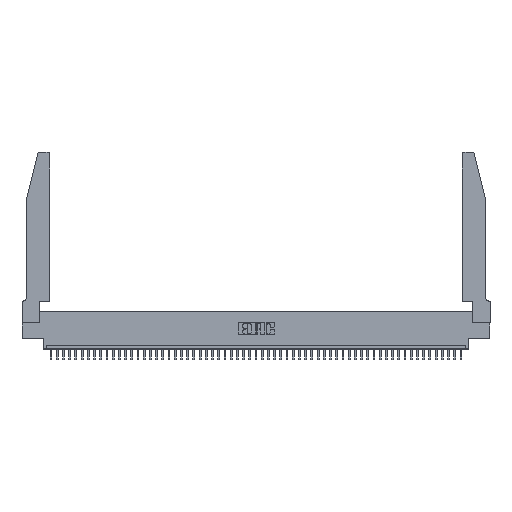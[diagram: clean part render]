
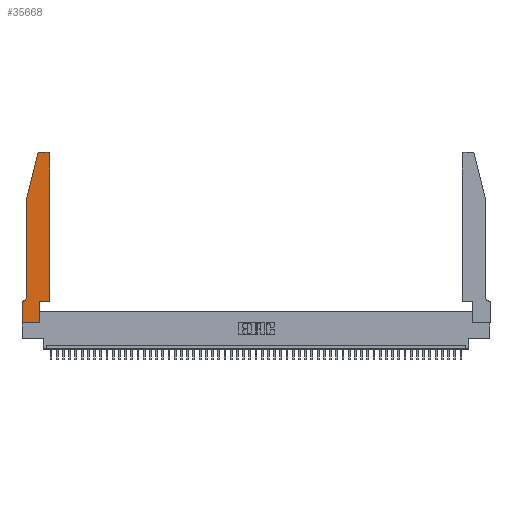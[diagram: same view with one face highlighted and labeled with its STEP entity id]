
A CAD part, top view. The second image highlights one B-rep face of the part: STEP entity #35668.
In plain terms, the highlighted planar face has unit normal (0, 0, 1).
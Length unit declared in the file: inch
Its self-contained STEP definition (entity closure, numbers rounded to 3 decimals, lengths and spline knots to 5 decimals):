
#62 = ORIENTED_EDGE ( 'NONE', *, *, #50955, .T. ) ;
#343 = CARTESIAN_POINT ( 'NONE',  ( 0., 0., 0.37 ) ) ;
#1142 = EDGE_CURVE ( 'NONE', #28846, #50141, #6747, .T. ) ;
#1306 = EDGE_CURVE ( 'NONE', #29648, #46651, #25623, .T. ) ;
#2280 = DIRECTION ( 'NONE',  ( 1., 0., 0. ) ) ;
#3753 = FACE_OUTER_BOUND ( 'NONE', #46519, .T. ) ;
#3962 = CIRCLE ( 'NONE', #47145, 0.03 ) ;
#3982 = VERTEX_POINT ( 'NONE', #46699 ) ;
#6747 = CIRCLE ( 'NONE', #12762, 0.03 ) ;
#7330 = CARTESIAN_POINT ( 'NONE',  ( 0., 0., 0.37 ) ) ;
#8298 = ORIENTED_EDGE ( 'NONE', *, *, #42074, .T. ) ;
#8563 = ORIENTED_EDGE ( 'NONE', *, *, #1142, .T. ) ;
#8738 = CARTESIAN_POINT ( 'NONE',  ( 0.2605, 2.75, 0.37 ) ) ;
#8767 = ORIENTED_EDGE ( 'NONE', *, *, #27100, .T. ) ;
#9578 = VERTEX_POINT ( 'NONE', #15384 ) ;
#11108 = DIRECTION ( 'NONE',  ( 1., 0., 0. ) ) ;
#11119 = EDGE_CURVE ( 'NONE', #50141, #13274, #48692, .T. ) ;
#11511 = LINE ( 'NONE', #23959, #41728 ) ;
#12290 = DIRECTION ( 'NONE',  ( -1., 0., 0. ) ) ;
#12762 = AXIS2_PLACEMENT_3D ( 'NONE', #36238, #41979, #51217 ) ;
#13274 = VERTEX_POINT ( 'NONE', #37834 ) ;
#14535 = VERTEX_POINT ( 'NONE', #47477 ) ;
#15041 = VERTEX_POINT ( 'NONE', #45383 ) ;
#15384 = CARTESIAN_POINT ( 'NONE',  ( 0.4505, 0.35, 0.37 ) ) ;
#20037 = EDGE_CURVE ( 'NONE', #3982, #22525, #39281, .T. ) ;
#20119 = EDGE_CURVE ( 'NONE', #46651, #24187, #45483, .T. ) ;
#20615 = CARTESIAN_POINT ( 'NONE',  ( 0., 0.35, 0.37 ) ) ;
#21022 = ORIENTED_EDGE ( 'NONE', *, *, #22215, .T. ) ;
#21277 = CIRCLE ( 'NONE', #25380, 0.07 ) ;
#21805 = CARTESIAN_POINT ( 'NONE',  ( 0.0755, 2., 0.37 ) ) ;
#22215 = EDGE_CURVE ( 'NONE', #13274, #3982, #3962, .T. ) ;
#22328 = VECTOR ( 'NONE', #12290, 39.37008 ) ;
#22525 = VERTEX_POINT ( 'NONE', #51980 ) ;
#22927 = VECTOR ( 'NONE', #51286, 39.37008 ) ;
#23067 = VECTOR ( 'NONE', #24706, 39.37008 ) ;
#23182 = ORIENTED_EDGE ( 'NONE', *, *, #34098, .T. ) ;
#23959 = CARTESIAN_POINT ( 'NONE',  ( 0.0755, 2., 0.37 ) ) ;
#24187 = VERTEX_POINT ( 'NONE', #28839 ) ;
#24706 = DIRECTION ( 'NONE',  ( 0., 1., 0. ) ) ;
#25380 = AXIS2_PLACEMENT_3D ( 'NONE', #26787, #30140, #29959 ) ;
#25623 = LINE ( 'NONE', #343, #45093 ) ;
#25815 = EDGE_CURVE ( 'NONE', #14535, #51537, #21277, .T. ) ;
#25866 = DIRECTION ( 'NONE',  ( -0.239, -0.971, 0. ) ) ;
#26787 = CARTESIAN_POINT ( 'NONE',  ( 0.0055, 0.42, 0.37 ) ) ;
#27100 = EDGE_CURVE ( 'NONE', #24187, #15041, #36290, .T. ) ;
#27217 = CARTESIAN_POINT ( 'NONE',  ( 0.284, 2.72, 0.37 ) ) ;
#27806 = CARTESIAN_POINT ( 'NONE',  ( 0.0755, 0.35, 0.37 ) ) ;
#28839 = CARTESIAN_POINT ( 'NONE',  ( 0.2865, 0., 0.37 ) ) ;
#28846 = VERTEX_POINT ( 'NONE', #49686 ) ;
#29423 = AXIS2_PLACEMENT_3D ( 'NONE', #49672, #49499, #49326 ) ;
#29565 = DIRECTION ( 'NONE',  ( 0., 1., 0. ) ) ;
#29648 = VERTEX_POINT ( 'NONE', #20615 ) ;
#29959 = DIRECTION ( 'NONE',  ( -1., 0., 0. ) ) ;
#30140 = DIRECTION ( 'NONE',  ( 0., 0., -1. ) ) ;
#30960 = LINE ( 'NONE', #33437, #47206 ) ;
#31193 = VECTOR ( 'NONE', #31869, 39.37008 ) ;
#31809 = DIRECTION ( 'NONE',  ( 0., 0., 1. ) ) ;
#31869 = DIRECTION ( 'NONE',  ( -1., 0., 0. ) ) ;
#33437 = CARTESIAN_POINT ( 'NONE',  ( 0.4505, 0.35, 0.37 ) ) ;
#34098 = EDGE_CURVE ( 'NONE', #15041, #9578, #44808, .T. ) ;
#35580 = LINE ( 'NONE', #27806, #31193 ) ;
#35668 = ADVANCED_FACE ( 'NONE', ( #3753 ), #45289, .T. ) ;
#36238 = CARTESIAN_POINT ( 'NONE',  ( 0.4205, 2.72, 0.37 ) ) ;
#36290 = LINE ( 'NONE', #48574, #23067 ) ;
#37834 = CARTESIAN_POINT ( 'NONE',  ( 0.284, 2.75, 0.37 ) ) ;
#38508 = ORIENTED_EDGE ( 'NONE', *, *, #49783, .T. ) ;
#39200 = ORIENTED_EDGE ( 'NONE', *, *, #25815, .T. ) ;
#39281 = LINE ( 'NONE', #21805, #44243 ) ;
#39621 = DIRECTION ( 'NONE',  ( 0., -1., 0. ) ) ;
#40864 = ORIENTED_EDGE ( 'NONE', *, *, #20037, .T. ) ;
#41339 = ORIENTED_EDGE ( 'NONE', *, *, #1306, .T. ) ;
#41728 = VECTOR ( 'NONE', #39621, 39.37008 ) ;
#41979 = DIRECTION ( 'NONE',  ( 0., 0., 1. ) ) ;
#42074 = EDGE_CURVE ( 'NONE', #9578, #28846, #30960, .T. ) ;
#42295 = CARTESIAN_POINT ( 'NONE',  ( 0.4505, 0.35, 0.37 ) ) ;
#42935 = CARTESIAN_POINT ( 'NONE',  ( 0., 0., 0.37 ) ) ;
#43049 = ORIENTED_EDGE ( 'NONE', *, *, #20119, .T. ) ;
#44243 = VECTOR ( 'NONE', #25866, 39.37008 ) ;
#44808 = LINE ( 'NONE', #42295, #50422 ) ;
#44882 = DIRECTION ( 'NONE',  ( 0., -1., 0. ) ) ;
#45093 = VECTOR ( 'NONE', #44882, 39.37008 ) ;
#45289 = PLANE ( 'NONE',  #29423 ) ;
#45383 = CARTESIAN_POINT ( 'NONE',  ( 0.2865, 0.35, 0.37 ) ) ;
#45483 = LINE ( 'NONE', #42935, #22927 ) ;
#46519 = EDGE_LOOP ( 'NONE', ( #48832, #21022, #40864, #62, #39200, #38508, #41339, #43049, #8767, #23182, #8298, #8563 ) ) ;
#46651 = VERTEX_POINT ( 'NONE', #7330 ) ;
#46669 = CARTESIAN_POINT ( 'NONE',  ( 0.4205, 2.75, 0.37 ) ) ;
#46699 = CARTESIAN_POINT ( 'NONE',  ( 0.25487, 2.72718, 0.37 ) ) ;
#47145 = AXIS2_PLACEMENT_3D ( 'NONE', #27217, #31809, #11108 ) ;
#47206 = VECTOR ( 'NONE', #29565, 39.37008 ) ;
#47477 = CARTESIAN_POINT ( 'NONE',  ( 0.0755, 0.42, 0.37 ) ) ;
#48574 = CARTESIAN_POINT ( 'NONE',  ( 0.2865, 0.35, 0.37 ) ) ;
#48692 = LINE ( 'NONE', #8738, #22328 ) ;
#48832 = ORIENTED_EDGE ( 'NONE', *, *, #11119, .T. ) ;
#49326 = DIRECTION ( 'NONE',  ( 1., 0., 0. ) ) ;
#49499 = DIRECTION ( 'NONE',  ( 0., 0., 1. ) ) ;
#49672 = CARTESIAN_POINT ( 'NONE',  ( 0., 0.35, 0.37 ) ) ;
#49686 = CARTESIAN_POINT ( 'NONE',  ( 0.4505, 2.72, 0.37 ) ) ;
#49783 = EDGE_CURVE ( 'NONE', #51537, #29648, #35580, .T. ) ;
#50141 = VERTEX_POINT ( 'NONE', #46669 ) ;
#50422 = VECTOR ( 'NONE', #2280, 39.37008 ) ;
#50955 = EDGE_CURVE ( 'NONE', #22525, #14535, #11511, .T. ) ;
#51217 = DIRECTION ( 'NONE',  ( 1., 0., 0. ) ) ;
#51286 = DIRECTION ( 'NONE',  ( 1., 0., 0. ) ) ;
#51425 = CARTESIAN_POINT ( 'NONE',  ( 0.0055, 0.35, 0.37 ) ) ;
#51537 = VERTEX_POINT ( 'NONE', #51425 ) ;
#51980 = CARTESIAN_POINT ( 'NONE',  ( 0.0755, 2., 0.37 ) ) ;
